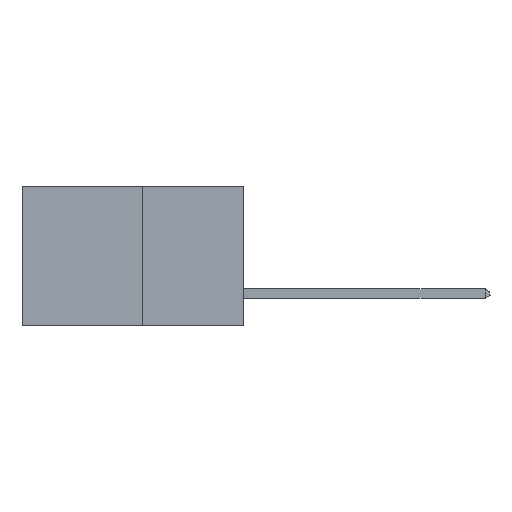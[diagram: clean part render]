
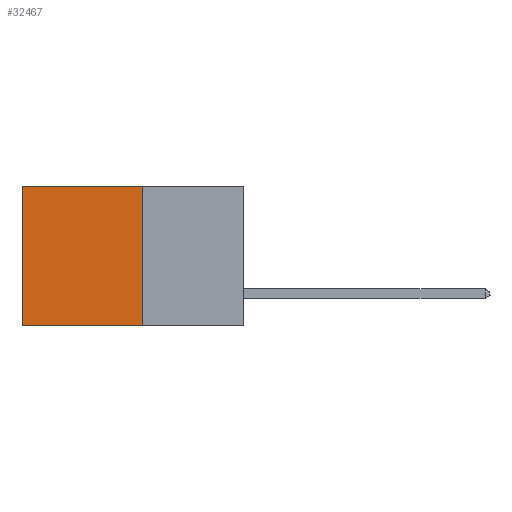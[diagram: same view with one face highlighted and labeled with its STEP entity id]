
A CAD part, left-side view. The second image highlights one B-rep face of the part: STEP entity #32467.
In plain terms, the highlighted planar face has unit normal (-1, 0, 0).
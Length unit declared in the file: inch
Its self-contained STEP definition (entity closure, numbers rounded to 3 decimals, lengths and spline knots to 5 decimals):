
#1085 = CARTESIAN_POINT ( 'NONE',  ( 0.277, 0.59, 0. ) ) ;
#2193 = EDGE_CURVE ( 'NONE', #17829, #5087, #7620, .T. ) ;
#4389 = ORIENTED_EDGE ( 'NONE', *, *, #21085, .T. ) ;
#4815 = DIRECTION ( 'NONE',  ( 0., 1., 0. ) ) ;
#5087 = VERTEX_POINT ( 'NONE', #11328 ) ;
#5187 = CARTESIAN_POINT ( 'NONE',  ( 0.277, 0.27, -0.37 ) ) ;
#6791 = VECTOR ( 'NONE', #4815, 39.37008 ) ;
#6815 = CARTESIAN_POINT ( 'NONE',  ( 0.277, 0.27, -0.37 ) ) ;
#7478 = VECTOR ( 'NONE', #12019, 39.37008 ) ;
#7620 = LINE ( 'NONE', #5187, #6791 ) ;
#8244 = ORIENTED_EDGE ( 'NONE', *, *, #32367, .F. ) ;
#8418 = CARTESIAN_POINT ( 'NONE',  ( 0.277, 0.59, -0.37 ) ) ;
#9488 = DIRECTION ( 'NONE',  ( 1., 0., 0. ) ) ;
#9633 = LINE ( 'NONE', #8418, #29695 ) ;
#11328 = CARTESIAN_POINT ( 'NONE',  ( 0.277, 0.59, -0.37 ) ) ;
#12019 = DIRECTION ( 'NONE',  ( 0., 1., 0. ) ) ;
#14539 = LINE ( 'NONE', #25150, #7478 ) ;
#14784 = VECTOR ( 'NONE', #22290, 39.37008 ) ;
#16413 = DIRECTION ( 'NONE',  ( 0., 0., -1. ) ) ;
#17829 = VERTEX_POINT ( 'NONE', #30447 ) ;
#18360 = EDGE_CURVE ( 'NONE', #33889, #24270, #14539, .T. ) ;
#19651 = AXIS2_PLACEMENT_3D ( 'NONE', #6815, #9488, #27816 ) ;
#21085 = EDGE_CURVE ( 'NONE', #24270, #5087, #9633, .T. ) ;
#21755 = ORIENTED_EDGE ( 'NONE', *, *, #18360, .T. ) ;
#22290 = DIRECTION ( 'NONE',  ( 0., 0., -1. ) ) ;
#24264 = ORIENTED_EDGE ( 'NONE', *, *, #2193, .F. ) ;
#24270 = VERTEX_POINT ( 'NONE', #1085 ) ;
#25150 = CARTESIAN_POINT ( 'NONE',  ( 0.277, 0.27, 0. ) ) ;
#25266 = PLANE ( 'NONE',  #19651 ) ;
#25471 = FACE_OUTER_BOUND ( 'NONE', #29175, .T. ) ;
#27816 = DIRECTION ( 'NONE',  ( 0., 0., -1. ) ) ;
#29175 = EDGE_LOOP ( 'NONE', ( #4389, #24264, #8244, #21755 ) ) ;
#29465 = LINE ( 'NONE', #29980, #14784 ) ;
#29695 = VECTOR ( 'NONE', #16413, 39.37008 ) ;
#29980 = CARTESIAN_POINT ( 'NONE',  ( 0.277, 0.27, -0.37 ) ) ;
#30447 = CARTESIAN_POINT ( 'NONE',  ( 0.277, 0.27, -0.37 ) ) ;
#32367 = EDGE_CURVE ( 'NONE', #33889, #17829, #29465, .T. ) ;
#32467 = ADVANCED_FACE ( 'NONE', ( #25471 ), #25266, .F. ) ;
#33359 = CARTESIAN_POINT ( 'NONE',  ( 0.277, 0.27, 0. ) ) ;
#33889 = VERTEX_POINT ( 'NONE', #33359 ) ;
